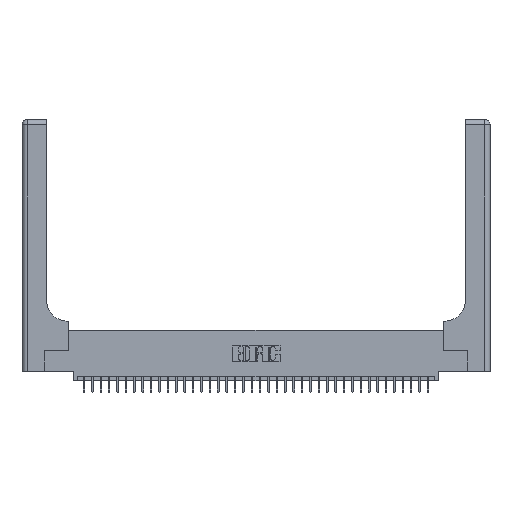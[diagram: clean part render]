
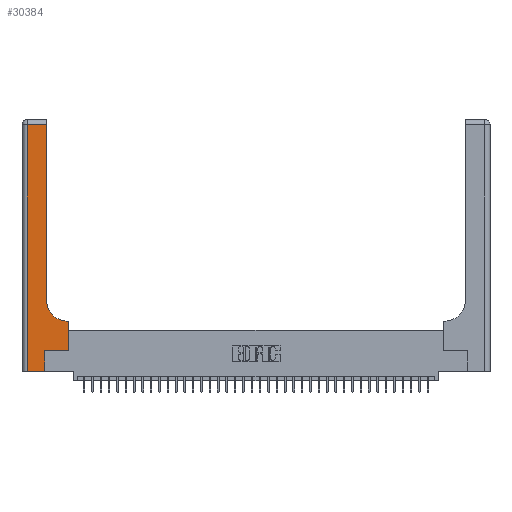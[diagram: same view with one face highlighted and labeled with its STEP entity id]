
A CAD part, top view. The second image highlights one B-rep face of the part: STEP entity #30384.
In plain terms, the highlighted planar face has unit normal (0, 0, 1).
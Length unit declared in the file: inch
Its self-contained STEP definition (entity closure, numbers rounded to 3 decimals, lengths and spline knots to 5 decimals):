
#53 = DIRECTION ( 'NONE',  ( -1., 0., 0. ) ) ;
#737 = CARTESIAN_POINT ( 'NONE',  ( 0.06, 0., 0.37 ) ) ;
#1443 = LINE ( 'NONE', #25174, #24527 ) ;
#2996 = ORIENTED_EDGE ( 'NONE', *, *, #7705, .T. ) ;
#3084 = ORIENTED_EDGE ( 'NONE', *, *, #21721, .T. ) ;
#3291 = LINE ( 'NONE', #15167, #26764 ) ;
#3634 = VERTEX_POINT ( 'NONE', #18920 ) ;
#4046 = VECTOR ( 'NONE', #32467, 39.37008 ) ;
#4655 = DIRECTION ( 'NONE',  ( 0., 1., 0. ) ) ;
#4806 = CARTESIAN_POINT ( 'NONE',  ( 0.5415, 0.6, 0.37 ) ) ;
#5219 = LINE ( 'NONE', #28534, #17831 ) ;
#6229 = CARTESIAN_POINT ( 'NONE',  ( 0.269, 0.25, 0.37 ) ) ;
#6514 = CARTESIAN_POINT ( 'NONE',  ( 0.2915, 0.85, 0.37 ) ) ;
#6697 = DIRECTION ( 'NONE',  ( -1., 0., 0. ) ) ;
#7140 = CARTESIAN_POINT ( 'NONE',  ( 0.5585, 0.6, 0.37 ) ) ;
#7705 = EDGE_CURVE ( 'NONE', #9650, #32660, #1443, .T. ) ;
#7798 = FACE_OUTER_BOUND ( 'NONE', #19734, .T. ) ;
#7942 = ORIENTED_EDGE ( 'NONE', *, *, #13147, .T. ) ;
#7992 = DIRECTION ( 'NONE',  ( -1., 0., 0. ) ) ;
#8070 = ORIENTED_EDGE ( 'NONE', *, *, #36767, .T. ) ;
#8976 = LINE ( 'NONE', #20839, #4046 ) ;
#9650 = VERTEX_POINT ( 'NONE', #6514 ) ;
#10001 = CARTESIAN_POINT ( 'NONE',  ( 0., 2.94, 0.37 ) ) ;
#10193 = CARTESIAN_POINT ( 'NONE',  ( 0.5415, 0.85, 0.37 ) ) ;
#10359 = VERTEX_POINT ( 'NONE', #19989 ) ;
#10363 = EDGE_CURVE ( 'NONE', #10359, #17483, #5219, .T. ) ;
#10608 = VERTEX_POINT ( 'NONE', #7140 ) ;
#11506 = VECTOR ( 'NONE', #6697, 39.37008 ) ;
#13147 = EDGE_CURVE ( 'NONE', #32660, #23066, #36592, .T. ) ;
#13934 = LINE ( 'NONE', #16473, #28881 ) ;
#13979 = CARTESIAN_POINT ( 'NONE',  ( 0.06, 2.94, 0.37 ) ) ;
#15167 = CARTESIAN_POINT ( 'NONE',  ( 0., 0., 0.37 ) ) ;
#16358 = CARTESIAN_POINT ( 'NONE',  ( 0., 3., 0.37 ) ) ;
#16473 = CARTESIAN_POINT ( 'NONE',  ( 0.06, 3., 0.37 ) ) ;
#16544 = DIRECTION ( 'NONE',  ( 1., 0., 0. ) ) ;
#17483 = VERTEX_POINT ( 'NONE', #6229 ) ;
#17831 = VECTOR ( 'NONE', #4655, 39.37008 ) ;
#18172 = CARTESIAN_POINT ( 'NONE',  ( 0.2915, 2.94, 0.37 ) ) ;
#18920 = CARTESIAN_POINT ( 'NONE',  ( 0.5585, 0.25, 0.37 ) ) ;
#19449 = VECTOR ( 'NONE', #53, 39.37008 ) ;
#19734 = EDGE_LOOP ( 'NONE', ( #2996, #7942, #35191, #3084, #33756, #34246, #8070, #25655, #35140 ) ) ;
#19768 = DIRECTION ( 'NONE',  ( 0., -1., 0. ) ) ;
#19989 = CARTESIAN_POINT ( 'NONE',  ( 0.269, 0., 0.37 ) ) ;
#20647 = CARTESIAN_POINT ( 'NONE',  ( 0.2915, 0.6, 0.37 ) ) ;
#20839 = CARTESIAN_POINT ( 'NONE',  ( 0.5585, 0.25, 0.37 ) ) ;
#21485 = DIRECTION ( 'NONE',  ( 1., 0., 0. ) ) ;
#21721 = EDGE_CURVE ( 'NONE', #34063, #10359, #3291, .T. ) ;
#23066 = VERTEX_POINT ( 'NONE', #13979 ) ;
#23417 = VERTEX_POINT ( 'NONE', #4806 ) ;
#23752 = LINE ( 'NONE', #20647, #19449 ) ;
#24527 = VECTOR ( 'NONE', #25541, 39.37008 ) ;
#25174 = CARTESIAN_POINT ( 'NONE',  ( 0.2915, 3., 0.37 ) ) ;
#25426 = EDGE_CURVE ( 'NONE', #23417, #9650, #31210, .T. ) ;
#25541 = DIRECTION ( 'NONE',  ( 0., 1., 0. ) ) ;
#25655 = ORIENTED_EDGE ( 'NONE', *, *, #25686, .T. ) ;
#25686 = EDGE_CURVE ( 'NONE', #10608, #23417, #23752, .T. ) ;
#26764 = VECTOR ( 'NONE', #29905, 39.37008 ) ;
#28264 = EDGE_CURVE ( 'NONE', #23066, #34063, #13934, .T. ) ;
#28534 = CARTESIAN_POINT ( 'NONE',  ( 0.269, 0., 0.37 ) ) ;
#28709 = AXIS2_PLACEMENT_3D ( 'NONE', #10193, #33880, #21485 ) ;
#28881 = VECTOR ( 'NONE', #19768, 39.37008 ) ;
#29905 = DIRECTION ( 'NONE',  ( 1., 0., 0. ) ) ;
#30217 = AXIS2_PLACEMENT_3D ( 'NONE', #16358, #33831, #7992 ) ;
#30384 = ADVANCED_FACE ( 'NONE', ( #7798 ), #31105, .F. ) ;
#31105 = PLANE ( 'NONE',  #30217 ) ;
#31210 = CIRCLE ( 'NONE', #28709, 0.25 ) ;
#31482 = CARTESIAN_POINT ( 'NONE',  ( 0.269, 0.25, 0.37 ) ) ;
#31669 = LINE ( 'NONE', #31482, #33115 ) ;
#32467 = DIRECTION ( 'NONE',  ( 0., 1., 0. ) ) ;
#32660 = VERTEX_POINT ( 'NONE', #18172 ) ;
#33115 = VECTOR ( 'NONE', #16544, 39.37008 ) ;
#33756 = ORIENTED_EDGE ( 'NONE', *, *, #10363, .T. ) ;
#33831 = DIRECTION ( 'NONE',  ( 0., 0., -1. ) ) ;
#33880 = DIRECTION ( 'NONE',  ( 0., 0., -1. ) ) ;
#34063 = VERTEX_POINT ( 'NONE', #737 ) ;
#34246 = ORIENTED_EDGE ( 'NONE', *, *, #35679, .T. ) ;
#35140 = ORIENTED_EDGE ( 'NONE', *, *, #25426, .T. ) ;
#35191 = ORIENTED_EDGE ( 'NONE', *, *, #28264, .T. ) ;
#35679 = EDGE_CURVE ( 'NONE', #17483, #3634, #31669, .T. ) ;
#36592 = LINE ( 'NONE', #10001, #11506 ) ;
#36767 = EDGE_CURVE ( 'NONE', #3634, #10608, #8976, .T. ) ;
